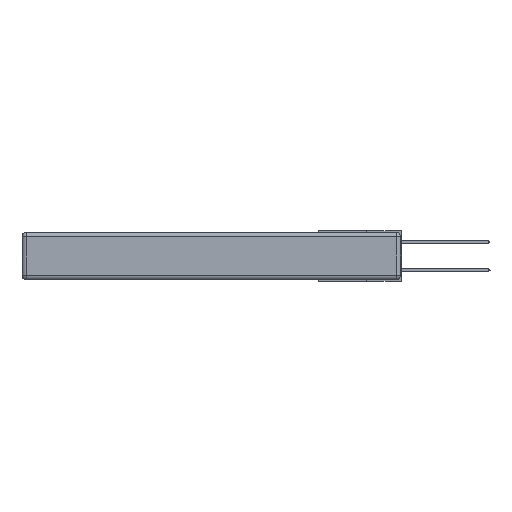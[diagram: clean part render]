
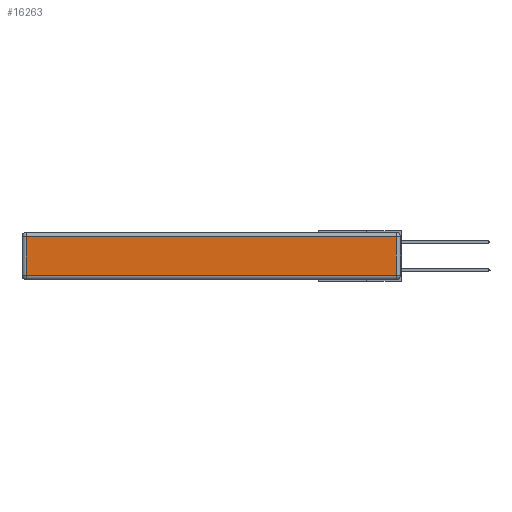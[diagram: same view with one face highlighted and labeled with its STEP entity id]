
A CAD part, left-side view. The second image highlights one B-rep face of the part: STEP entity #16263.
In plain terms, the highlighted planar face has unit normal (-1, 0, 0).
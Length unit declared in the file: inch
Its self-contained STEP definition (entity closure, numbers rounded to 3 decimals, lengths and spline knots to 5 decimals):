
#4183 = VERTEX_POINT ( 'NONE', #6659 ) ;
#6367 = VECTOR ( 'NONE', #27181, 39.37008 ) ;
#6541 = ORIENTED_EDGE ( 'NONE', *, *, #26250, .T. ) ;
#6659 = CARTESIAN_POINT ( 'NONE',  ( 0., 2.72, -0.03 ) ) ;
#7076 = DIRECTION ( 'NONE',  ( -1., 0., 0. ) ) ;
#7162 = VERTEX_POINT ( 'NONE', #11473 ) ;
#8334 = CARTESIAN_POINT ( 'NONE',  ( 0., 0.03, -0.343 ) ) ;
#8668 = EDGE_CURVE ( 'NONE', #20953, #4183, #13515, .T. ) ;
#8768 = AXIS2_PLACEMENT_3D ( 'NONE', #18116, #7076, #22396 ) ;
#11055 = EDGE_LOOP ( 'NONE', ( #16365, #19797, #28873, #6541 ) ) ;
#11473 = CARTESIAN_POINT ( 'NONE',  ( 0., 2.72, -0.313 ) ) ;
#12084 = CARTESIAN_POINT ( 'NONE',  ( 0., 0.03, -0.313 ) ) ;
#12290 = LINE ( 'NONE', #24879, #6367 ) ;
#12322 = EDGE_CURVE ( 'NONE', #20918, #20953, #21936, .T. ) ;
#13515 = LINE ( 'NONE', #27501, #28210 ) ;
#14420 = CARTESIAN_POINT ( 'NONE',  ( 0., 0.03, -0.03 ) ) ;
#15695 = VECTOR ( 'NONE', #23873, 39.37008 ) ;
#16019 = DIRECTION ( 'NONE',  ( 0., 0., -1. ) ) ;
#16263 = ADVANCED_FACE ( 'NONE', ( #16845 ), #26967, .T. ) ;
#16365 = ORIENTED_EDGE ( 'NONE', *, *, #22610, .T. ) ;
#16845 = FACE_OUTER_BOUND ( 'NONE', #11055, .T. ) ;
#17988 = CARTESIAN_POINT ( 'NONE',  ( 0., 2.72, -0.343 ) ) ;
#18116 = CARTESIAN_POINT ( 'NONE',  ( 0., 0., -0.343 ) ) ;
#19797 = ORIENTED_EDGE ( 'NONE', *, *, #12322, .T. ) ;
#20918 = VERTEX_POINT ( 'NONE', #12084 ) ;
#20953 = VERTEX_POINT ( 'NONE', #14420 ) ;
#21936 = LINE ( 'NONE', #8334, #15695 ) ;
#22396 = DIRECTION ( 'NONE',  ( 0., 0., 1. ) ) ;
#22610 = EDGE_CURVE ( 'NONE', #7162, #20918, #12290, .T. ) ;
#22828 = DIRECTION ( 'NONE',  ( 0., 1., 0. ) ) ;
#23171 = LINE ( 'NONE', #17988, #23889 ) ;
#23873 = DIRECTION ( 'NONE',  ( 0., 0., 1. ) ) ;
#23889 = VECTOR ( 'NONE', #16019, 39.37008 ) ;
#24879 = CARTESIAN_POINT ( 'NONE',  ( 0., 0., -0.313 ) ) ;
#26250 = EDGE_CURVE ( 'NONE', #4183, #7162, #23171, .T. ) ;
#26967 = PLANE ( 'NONE',  #8768 ) ;
#27181 = DIRECTION ( 'NONE',  ( 0., -1., 0. ) ) ;
#27501 = CARTESIAN_POINT ( 'NONE',  ( 0., 2.75, -0.03 ) ) ;
#28210 = VECTOR ( 'NONE', #22828, 39.37008 ) ;
#28873 = ORIENTED_EDGE ( 'NONE', *, *, #8668, .T. ) ;
